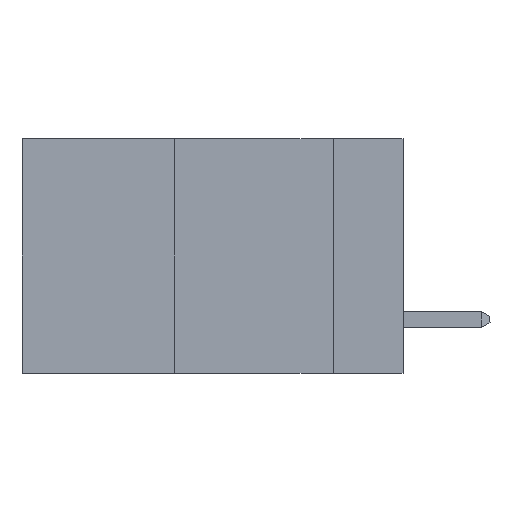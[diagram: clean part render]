
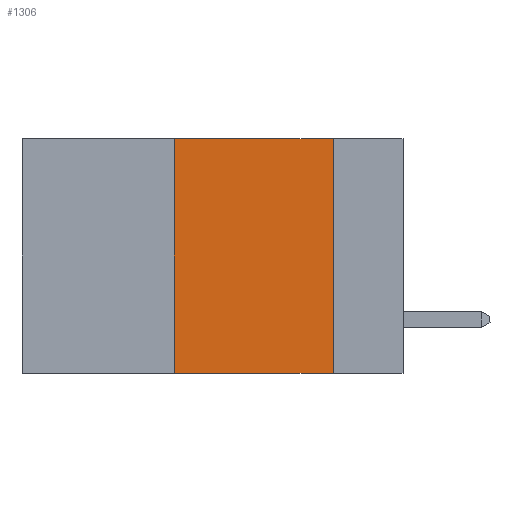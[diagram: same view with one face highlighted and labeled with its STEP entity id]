
A CAD part, left-side view. The second image highlights one B-rep face of the part: STEP entity #1306.
In plain terms, the highlighted planar face has unit normal (-1, 0, 0).
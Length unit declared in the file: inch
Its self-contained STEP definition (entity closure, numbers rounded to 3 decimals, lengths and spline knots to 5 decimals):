
#32 = CARTESIAN_POINT ( 'NONE',  ( 0., 0.11, -0.37 ) ) ;
#245 = EDGE_LOOP ( 'NONE', ( #1527, #1577, #1594, #1649 ) ) ;
#546 = CARTESIAN_POINT ( 'NONE',  ( 0., 0.11, 0. ) ) ;
#894 = LINE ( 'NONE', #4760, #5645 ) ;
#1306 = ADVANCED_FACE ( 'NONE', ( #7855 ), #4534, .F. ) ;
#1527 = ORIENTED_EDGE ( 'NONE', *, *, #1756, .F. ) ;
#1577 = ORIENTED_EDGE ( 'NONE', *, *, #10713, .F. ) ;
#1594 = ORIENTED_EDGE ( 'NONE', *, *, #3471, .F. ) ;
#1617 = VERTEX_POINT ( 'NONE', #32 ) ;
#1649 = ORIENTED_EDGE ( 'NONE', *, *, #10586, .T. ) ;
#1756 = EDGE_CURVE ( 'NONE', #4125, #1617, #9766, .T. ) ;
#2454 = CARTESIAN_POINT ( 'NONE',  ( 0., 0.36, 0. ) ) ;
#2478 = DIRECTION ( 'NONE',  ( 0., 0., 1. ) ) ;
#3471 = EDGE_CURVE ( 'NONE', #7645, #8992, #7934, .T. ) ;
#3509 = CARTESIAN_POINT ( 'NONE',  ( 0., 0.36, 0. ) ) ;
#4125 = VERTEX_POINT ( 'NONE', #546 ) ;
#4265 = LINE ( 'NONE', #8887, #10468 ) ;
#4515 = DIRECTION ( 'NONE',  ( 0., 0., -1. ) ) ;
#4522 = DIRECTION ( 'NONE',  ( 1., 0., 0. ) ) ;
#4534 = PLANE ( 'NONE',  #6109 ) ;
#4760 = CARTESIAN_POINT ( 'NONE',  ( 0., 0.6, -0.37 ) ) ;
#4773 = CARTESIAN_POINT ( 'NONE',  ( 0., 0.6, 0. ) ) ;
#4934 = DIRECTION ( 'NONE',  ( 0., -1., 0. ) ) ;
#5000 = VECTOR ( 'NONE', #2478, 39.37008 ) ;
#5358 = CARTESIAN_POINT ( 'NONE',  ( 0., 0.11, 0. ) ) ;
#5645 = VECTOR ( 'NONE', #6399, 39.37008 ) ;
#6109 = AXIS2_PLACEMENT_3D ( 'NONE', #4773, #4522, #4515 ) ;
#6399 = DIRECTION ( 'NONE',  ( 0., -1., 0. ) ) ;
#6856 = DIRECTION ( 'NONE',  ( 0., 0., -1. ) ) ;
#7645 = VERTEX_POINT ( 'NONE', #8078 ) ;
#7846 = VECTOR ( 'NONE', #6856, 39.37008 ) ;
#7855 = FACE_OUTER_BOUND ( 'NONE', #245, .T. ) ;
#7934 = LINE ( 'NONE', #2454, #5000 ) ;
#8078 = CARTESIAN_POINT ( 'NONE',  ( 0., 0.36, -0.37 ) ) ;
#8887 = CARTESIAN_POINT ( 'NONE',  ( 0., 0.6, 0. ) ) ;
#8992 = VERTEX_POINT ( 'NONE', #3509 ) ;
#9766 = LINE ( 'NONE', #5358, #7846 ) ;
#10468 = VECTOR ( 'NONE', #4934, 39.37008 ) ;
#10586 = EDGE_CURVE ( 'NONE', #7645, #1617, #894, .T. ) ;
#10713 = EDGE_CURVE ( 'NONE', #8992, #4125, #4265, .T. ) ;
